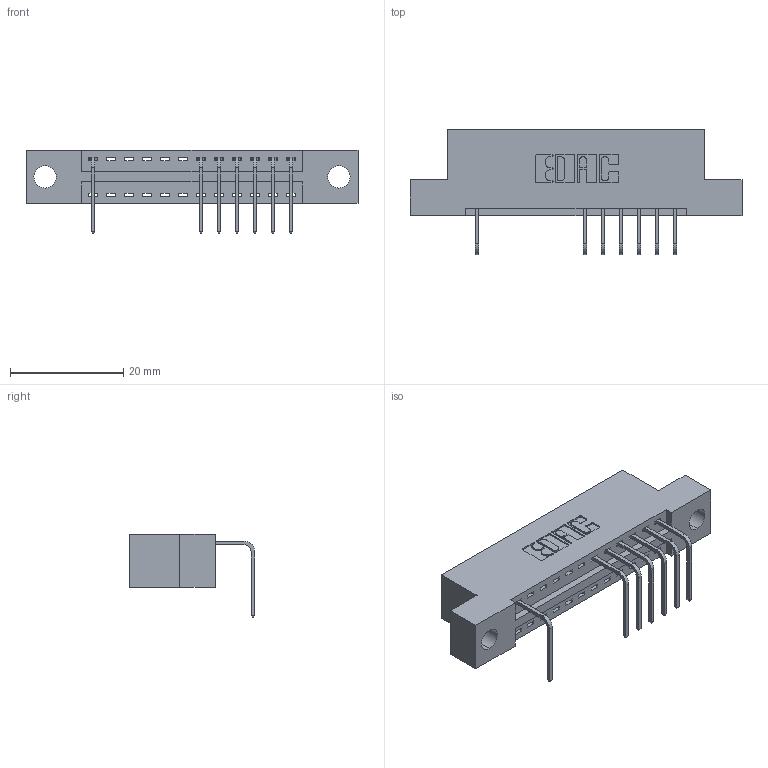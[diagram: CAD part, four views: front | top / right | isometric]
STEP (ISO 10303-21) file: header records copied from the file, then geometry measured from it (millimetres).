
FILE_DESCRIPTION (( 'STEP AP203' ), '1' );
FILE_NAME ('346-012-558-104.STEP', '2018-08-19T22:58:10', ( '' ), ( '' ), 'SwSTEP 2.0', 'SolidWorks 2016', '' );
FILE_SCHEMA (( 'CONFIG_CONTROL_DESIGN' ));
Length unit declared in the file: inch
Products named in the file (3): 346-012-558-104; 346 Part_Flush Mounting Lugs - 0.156 Dia-TH; 345-292-001_558 Tail - 2
Assembly tree (8 placements, depth 2):
  346-012-558-104
    346 Part_Flush Mounting Lugs - 0.156 Dia-TH
    345-292-001_558 Tail - 2  x7
Bounding box: 58.67 x 22.16 x 14.73 mm (x, y, z)
Volume: 5288 mm3; surface area: 5922 mm2
Topology: 8 solids, 8 shells, 602 faces, 1813 edges, 1198 vertices
Faces by surface type: plane 420, cylinder 182
Entity records: 11413 total; most frequent: CARTESIAN_POINT 1995, ORIENTED_EDGE 1946, DIRECTION 1791, EDGE_CURVE 973, LINE 793, VECTOR 793, VERTEX_POINT 646, AXIS2_PLACEMENT_3D 499
